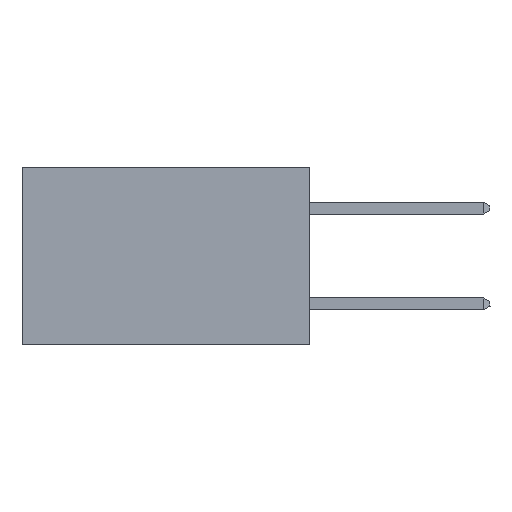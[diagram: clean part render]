
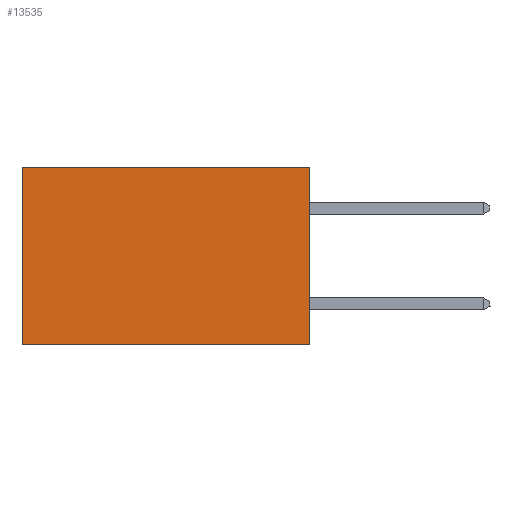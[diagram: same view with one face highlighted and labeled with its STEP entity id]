
A CAD part, left-side view. The second image highlights one B-rep face of the part: STEP entity #13535.
In plain terms, the highlighted planar face has unit normal (-1, 0, 0).
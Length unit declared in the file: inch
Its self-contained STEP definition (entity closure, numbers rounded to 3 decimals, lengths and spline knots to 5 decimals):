
#666 = EDGE_LOOP ( 'NONE', ( #1385, #9147, #6877, #7571 ) ) ;
#1385 = ORIENTED_EDGE ( 'NONE', *, *, #5270, .T. ) ;
#1668 = VECTOR ( 'NONE', #13532, 39.37008 ) ;
#2595 = CARTESIAN_POINT ( 'NONE',  ( 0.2875, 0., 0. ) ) ;
#3524 = LINE ( 'NONE', #5206, #10308 ) ;
#3589 = LINE ( 'NONE', #13495, #12520 ) ;
#3680 = CARTESIAN_POINT ( 'NONE',  ( 0.2875, 0.6, 0. ) ) ;
#4073 = CARTESIAN_POINT ( 'NONE',  ( 0.2875, 0.6, 0. ) ) ;
#4796 = AXIS2_PLACEMENT_3D ( 'NONE', #5612, #15621, #8157 ) ;
#5206 = CARTESIAN_POINT ( 'NONE',  ( 0.2875, 0., 0. ) ) ;
#5270 = EDGE_CURVE ( 'NONE', #10994, #5980, #9741, .T. ) ;
#5612 = CARTESIAN_POINT ( 'NONE',  ( 0.2875, 0., 0. ) ) ;
#5980 = VERTEX_POINT ( 'NONE', #13577 ) ;
#6361 = VECTOR ( 'NONE', #9473, 39.37008 ) ;
#6877 = ORIENTED_EDGE ( 'NONE', *, *, #13741, .F. ) ;
#7571 = ORIENTED_EDGE ( 'NONE', *, *, #14621, .T. ) ;
#8157 = DIRECTION ( 'NONE',  ( 0., 0., -1. ) ) ;
#9147 = ORIENTED_EDGE ( 'NONE', *, *, #13062, .F. ) ;
#9473 = DIRECTION ( 'NONE',  ( 0., 0., -1. ) ) ;
#9741 = LINE ( 'NONE', #3680, #6361 ) ;
#10308 = VECTOR ( 'NONE', #11557, 39.37008 ) ;
#10868 = CARTESIAN_POINT ( 'NONE',  ( 0.2875, 0., -0.37 ) ) ;
#10994 = VERTEX_POINT ( 'NONE', #4073 ) ;
#11557 = DIRECTION ( 'NONE',  ( 0., 1., 0. ) ) ;
#11727 = FACE_OUTER_BOUND ( 'NONE', #666, .T. ) ;
#12305 = LINE ( 'NONE', #12317, #1668 ) ;
#12317 = CARTESIAN_POINT ( 'NONE',  ( 0.2875, 0., 0. ) ) ;
#12520 = VECTOR ( 'NONE', #15921, 39.37008 ) ;
#12966 = VERTEX_POINT ( 'NONE', #10868 ) ;
#13062 = EDGE_CURVE ( 'NONE', #12966, #5980, #3589, .T. ) ;
#13495 = CARTESIAN_POINT ( 'NONE',  ( 0.2875, 0., -0.37 ) ) ;
#13532 = DIRECTION ( 'NONE',  ( 0., 0., -1. ) ) ;
#13535 = ADVANCED_FACE ( 'NONE', ( #11727 ), #14395, .F. ) ;
#13577 = CARTESIAN_POINT ( 'NONE',  ( 0.2875, 0.6, -0.37 ) ) ;
#13741 = EDGE_CURVE ( 'NONE', #14001, #12966, #12305, .T. ) ;
#14001 = VERTEX_POINT ( 'NONE', #2595 ) ;
#14395 = PLANE ( 'NONE',  #4796 ) ;
#14621 = EDGE_CURVE ( 'NONE', #14001, #10994, #3524, .T. ) ;
#15621 = DIRECTION ( 'NONE',  ( 1., 0., 0. ) ) ;
#15921 = DIRECTION ( 'NONE',  ( 0., 1., 0. ) ) ;
